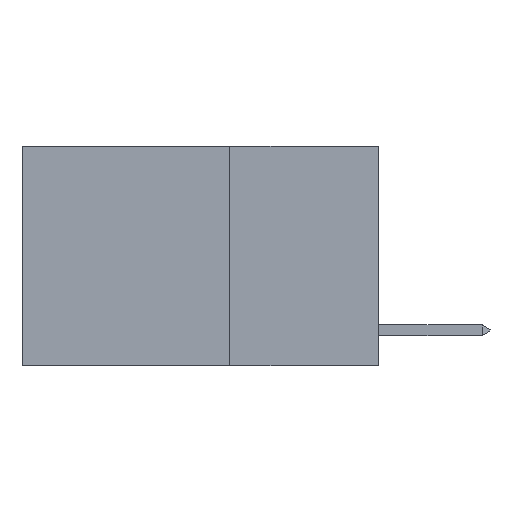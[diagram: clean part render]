
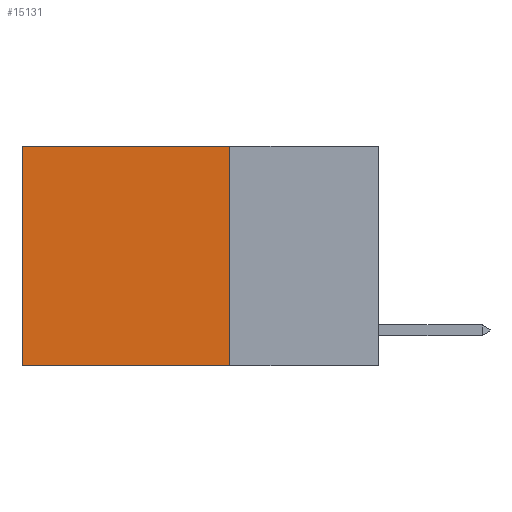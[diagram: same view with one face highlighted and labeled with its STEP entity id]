
A CAD part, left-side view. The second image highlights one B-rep face of the part: STEP entity #15131.
In plain terms, the highlighted planar face has unit normal (-1, 0, 0).
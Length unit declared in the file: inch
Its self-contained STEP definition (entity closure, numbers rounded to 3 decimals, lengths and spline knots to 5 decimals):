
#699 = VECTOR ( 'NONE', #13358, 39.37008 ) ;
#1648 = PLANE ( 'NONE',  #11840 ) ;
#2113 = DIRECTION ( 'NONE',  ( 0., 1., 0. ) ) ;
#2174 = CARTESIAN_POINT ( 'NONE',  ( 0.2625, 0.6, 0. ) ) ;
#2413 = LINE ( 'NONE', #12452, #13420 ) ;
#6089 = DIRECTION ( 'NONE',  ( 0., 0., -1. ) ) ;
#6220 = VERTEX_POINT ( 'NONE', #2174 ) ;
#7300 = EDGE_LOOP ( 'NONE', ( #16775, #13962, #20182, #23158 ) ) ;
#7722 = EDGE_CURVE ( 'NONE', #6220, #23710, #11549, .T. ) ;
#8657 = CARTESIAN_POINT ( 'NONE',  ( 0.2625, 0.6, 0. ) ) ;
#10979 = EDGE_CURVE ( 'NONE', #15231, #12319, #23176, .T. ) ;
#11109 = CARTESIAN_POINT ( 'NONE',  ( 0.2625, 0.6, -0.37 ) ) ;
#11549 = LINE ( 'NONE', #8657, #23042 ) ;
#11840 = AXIS2_PLACEMENT_3D ( 'NONE', #16956, #19145, #6089 ) ;
#12319 = VERTEX_POINT ( 'NONE', #24113 ) ;
#12452 = CARTESIAN_POINT ( 'NONE',  ( 0.2625, 0.25, 0. ) ) ;
#13358 = DIRECTION ( 'NONE',  ( 0., 0., -1. ) ) ;
#13420 = VECTOR ( 'NONE', #14633, 39.37008 ) ;
#13962 = ORIENTED_EDGE ( 'NONE', *, *, #18028, .F. ) ;
#14633 = DIRECTION ( 'NONE',  ( 0., 1., 0. ) ) ;
#15131 = ADVANCED_FACE ( 'NONE', ( #26046 ), #1648, .F. ) ;
#15231 = VERTEX_POINT ( 'NONE', #27919 ) ;
#15270 = CARTESIAN_POINT ( 'NONE',  ( 0.2625, 0.25, -0.37 ) ) ;
#16775 = ORIENTED_EDGE ( 'NONE', *, *, #7722, .T. ) ;
#16956 = CARTESIAN_POINT ( 'NONE',  ( 0.2625, 0.25, 0. ) ) ;
#18028 = EDGE_CURVE ( 'NONE', #12319, #23710, #23893, .T. ) ;
#19145 = DIRECTION ( 'NONE',  ( 1., 0., 0. ) ) ;
#20182 = ORIENTED_EDGE ( 'NONE', *, *, #10979, .F. ) ;
#21046 = EDGE_CURVE ( 'NONE', #15231, #6220, #2413, .T. ) ;
#21668 = DIRECTION ( 'NONE',  ( 0., 0., -1. ) ) ;
#23042 = VECTOR ( 'NONE', #21668, 39.37008 ) ;
#23158 = ORIENTED_EDGE ( 'NONE', *, *, #21046, .T. ) ;
#23176 = LINE ( 'NONE', #26240, #699 ) ;
#23710 = VERTEX_POINT ( 'NONE', #11109 ) ;
#23893 = LINE ( 'NONE', #15270, #24581 ) ;
#24113 = CARTESIAN_POINT ( 'NONE',  ( 0.2625, 0.25, -0.37 ) ) ;
#24581 = VECTOR ( 'NONE', #2113, 39.37008 ) ;
#26046 = FACE_OUTER_BOUND ( 'NONE', #7300, .T. ) ;
#26240 = CARTESIAN_POINT ( 'NONE',  ( 0.2625, 0.25, 0. ) ) ;
#27919 = CARTESIAN_POINT ( 'NONE',  ( 0.2625, 0.25, 0. ) ) ;
